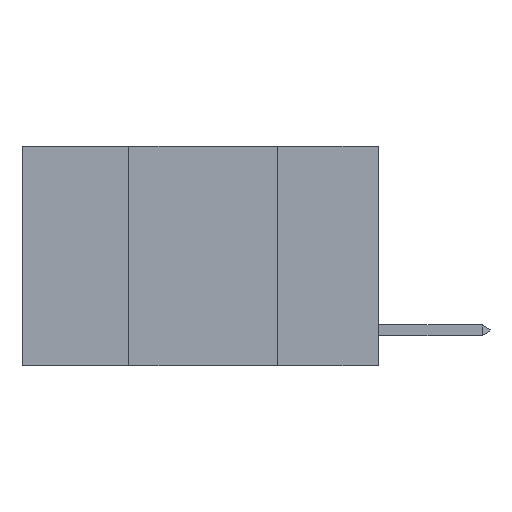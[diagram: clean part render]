
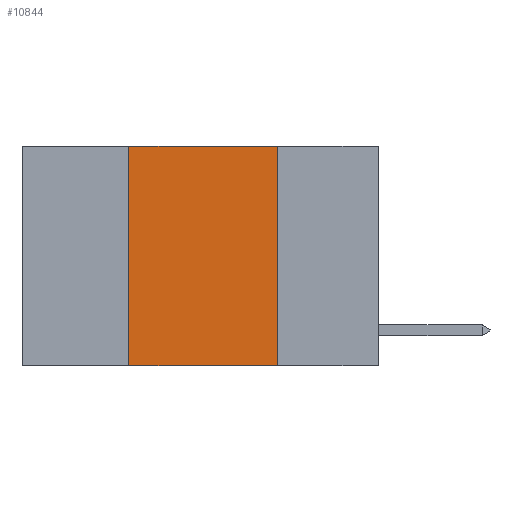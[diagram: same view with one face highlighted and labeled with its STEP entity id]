
A CAD part, left-side view. The second image highlights one B-rep face of the part: STEP entity #10844.
In plain terms, the highlighted planar face has unit normal (-1, 0, 0).
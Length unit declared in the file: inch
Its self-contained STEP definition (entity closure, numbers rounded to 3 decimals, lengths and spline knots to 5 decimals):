
#23 = VECTOR ( 'NONE', #4835, 39.37008 ) ;
#156 = CARTESIAN_POINT ( 'NONE',  ( 0., 0.17, -0.37 ) ) ;
#555 = DIRECTION ( 'NONE',  ( 0., -1., 0. ) ) ;
#997 = ORIENTED_EDGE ( 'NONE', *, *, #8893, .T. ) ;
#1081 = VERTEX_POINT ( 'NONE', #8207 ) ;
#1955 = ORIENTED_EDGE ( 'NONE', *, *, #4883, .F. ) ;
#2694 = LINE ( 'NONE', #9737, #11251 ) ;
#3128 = CARTESIAN_POINT ( 'NONE',  ( 0., 0.6, 0. ) ) ;
#3140 = EDGE_LOOP ( 'NONE', ( #4278, #1955, #6607, #997 ) ) ;
#3195 = CARTESIAN_POINT ( 'NONE',  ( 0., 0.6, -0.37 ) ) ;
#3965 = VECTOR ( 'NONE', #555, 39.37008 ) ;
#4130 = VERTEX_POINT ( 'NONE', #9277 ) ;
#4278 = ORIENTED_EDGE ( 'NONE', *, *, #10104, .F. ) ;
#4341 = VECTOR ( 'NONE', #10843, 39.37008 ) ;
#4366 = AXIS2_PLACEMENT_3D ( 'NONE', #3128, #10864, #5751 ) ;
#4835 = DIRECTION ( 'NONE',  ( 0., 0., 1. ) ) ;
#4883 = EDGE_CURVE ( 'NONE', #9352, #4130, #2694, .T. ) ;
#5724 = CARTESIAN_POINT ( 'NONE',  ( 0., 0.17, 0. ) ) ;
#5751 = DIRECTION ( 'NONE',  ( 0., 0., -1. ) ) ;
#6273 = LINE ( 'NONE', #3195, #3965 ) ;
#6607 = ORIENTED_EDGE ( 'NONE', *, *, #8832, .F. ) ;
#6797 = FACE_OUTER_BOUND ( 'NONE', #3140, .T. ) ;
#7243 = CARTESIAN_POINT ( 'NONE',  ( 0., 0.42, 0. ) ) ;
#8060 = VERTEX_POINT ( 'NONE', #156 ) ;
#8207 = CARTESIAN_POINT ( 'NONE',  ( 0., 0.42, -0.37 ) ) ;
#8832 = EDGE_CURVE ( 'NONE', #1081, #9352, #9384, .T. ) ;
#8893 = EDGE_CURVE ( 'NONE', #1081, #8060, #6273, .T. ) ;
#8949 = LINE ( 'NONE', #5724, #4341 ) ;
#9277 = CARTESIAN_POINT ( 'NONE',  ( 0., 0.17, 0. ) ) ;
#9352 = VERTEX_POINT ( 'NONE', #7243 ) ;
#9384 = LINE ( 'NONE', #10829, #23 ) ;
#9737 = CARTESIAN_POINT ( 'NONE',  ( 0., 0.6, 0. ) ) ;
#9772 = DIRECTION ( 'NONE',  ( 0., -1., 0. ) ) ;
#10039 = PLANE ( 'NONE',  #4366 ) ;
#10104 = EDGE_CURVE ( 'NONE', #4130, #8060, #8949, .T. ) ;
#10829 = CARTESIAN_POINT ( 'NONE',  ( 0., 0.42, 0. ) ) ;
#10843 = DIRECTION ( 'NONE',  ( 0., 0., -1. ) ) ;
#10844 = ADVANCED_FACE ( 'NONE', ( #6797 ), #10039, .F. ) ;
#10864 = DIRECTION ( 'NONE',  ( 1., 0., 0. ) ) ;
#11251 = VECTOR ( 'NONE', #9772, 39.37008 ) ;
